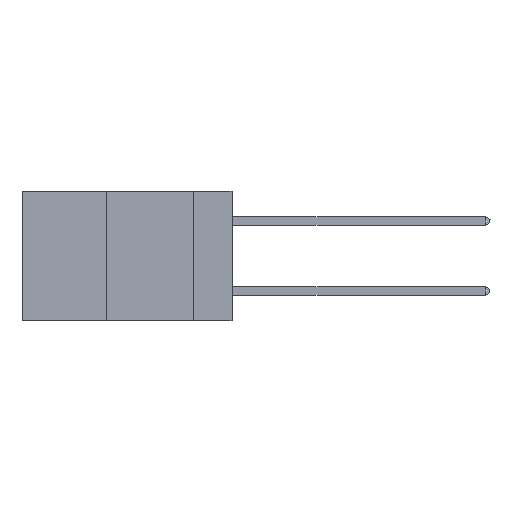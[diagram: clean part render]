
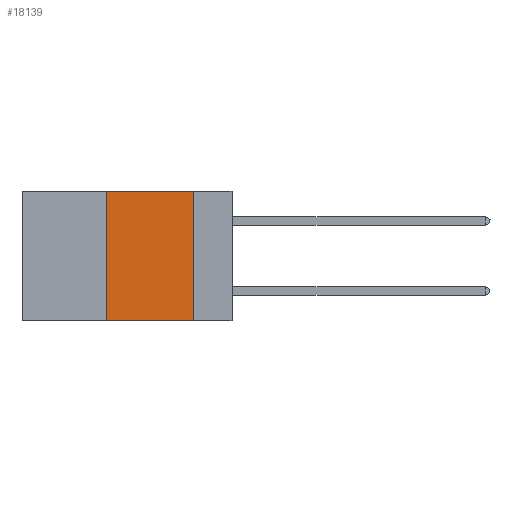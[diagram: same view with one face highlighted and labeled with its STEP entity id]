
A CAD part, left-side view. The second image highlights one B-rep face of the part: STEP entity #18139.
In plain terms, the highlighted planar face has unit normal (-1, 0, 0).
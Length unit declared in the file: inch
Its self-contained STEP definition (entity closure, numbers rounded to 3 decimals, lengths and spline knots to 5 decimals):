
#547 = VECTOR ( 'NONE', #659, 39.37008 ) ;
#659 = DIRECTION ( 'NONE',  ( 0., 0., 1. ) ) ;
#1109 = ORIENTED_EDGE ( 'NONE', *, *, #5071, .F. ) ;
#1276 = CARTESIAN_POINT ( 'NONE',  ( 0., 0.11, 0. ) ) ;
#1457 = PLANE ( 'NONE',  #12089 ) ;
#2424 = VERTEX_POINT ( 'NONE', #11779 ) ;
#2803 = LINE ( 'NONE', #14005, #17262 ) ;
#4216 = EDGE_CURVE ( 'NONE', #17185, #17579, #2803, .T. ) ;
#5071 = EDGE_CURVE ( 'NONE', #2424, #17185, #7564, .T. ) ;
#5444 = EDGE_CURVE ( 'NONE', #7664, #2424, #14556, .T. ) ;
#7258 = CARTESIAN_POINT ( 'NONE',  ( 0., 0.36, 0. ) ) ;
#7564 = LINE ( 'NONE', #17091, #14129 ) ;
#7664 = VERTEX_POINT ( 'NONE', #12804 ) ;
#8038 = ORIENTED_EDGE ( 'NONE', *, *, #4216, .F. ) ;
#8429 = EDGE_LOOP ( 'NONE', ( #8038, #1109, #16302, #13208 ) ) ;
#9446 = DIRECTION ( 'NONE',  ( 0., -1., 0. ) ) ;
#9716 = EDGE_CURVE ( 'NONE', #7664, #17579, #15745, .T. ) ;
#10155 = DIRECTION ( 'NONE',  ( 0., -1., 0. ) ) ;
#10476 = VECTOR ( 'NONE', #9446, 39.37008 ) ;
#11141 = DIRECTION ( 'NONE',  ( 1., 0., 0. ) ) ;
#11779 = CARTESIAN_POINT ( 'NONE',  ( 0., 0.36, 0. ) ) ;
#12089 = AXIS2_PLACEMENT_3D ( 'NONE', #12538, #11141, #13928 ) ;
#12129 = DIRECTION ( 'NONE',  ( 0., 0., -1. ) ) ;
#12538 = CARTESIAN_POINT ( 'NONE',  ( 0., 0.6, 0. ) ) ;
#12804 = CARTESIAN_POINT ( 'NONE',  ( 0., 0.36, -0.37 ) ) ;
#13208 = ORIENTED_EDGE ( 'NONE', *, *, #9716, .T. ) ;
#13928 = DIRECTION ( 'NONE',  ( 0., 0., -1. ) ) ;
#14005 = CARTESIAN_POINT ( 'NONE',  ( 0., 0.11, 0. ) ) ;
#14129 = VECTOR ( 'NONE', #10155, 39.37008 ) ;
#14556 = LINE ( 'NONE', #7258, #547 ) ;
#15399 = CARTESIAN_POINT ( 'NONE',  ( 0., 0.11, -0.37 ) ) ;
#15745 = LINE ( 'NONE', #16506, #10476 ) ;
#16302 = ORIENTED_EDGE ( 'NONE', *, *, #5444, .F. ) ;
#16506 = CARTESIAN_POINT ( 'NONE',  ( 0., 0.6, -0.37 ) ) ;
#17091 = CARTESIAN_POINT ( 'NONE',  ( 0., 0.6, 0. ) ) ;
#17179 = FACE_OUTER_BOUND ( 'NONE', #8429, .T. ) ;
#17185 = VERTEX_POINT ( 'NONE', #1276 ) ;
#17262 = VECTOR ( 'NONE', #12129, 39.37008 ) ;
#17579 = VERTEX_POINT ( 'NONE', #15399 ) ;
#18139 = ADVANCED_FACE ( 'NONE', ( #17179 ), #1457, .F. ) ;
